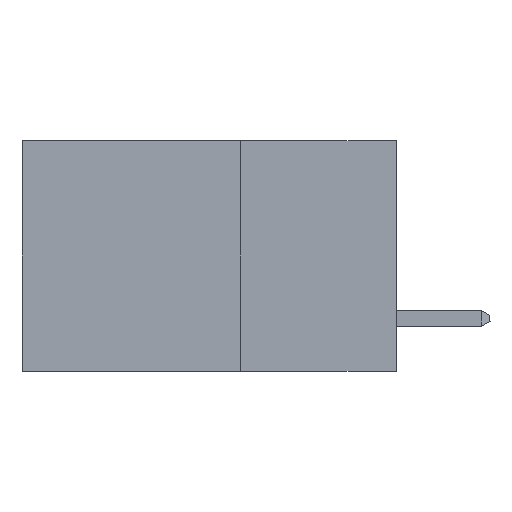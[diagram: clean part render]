
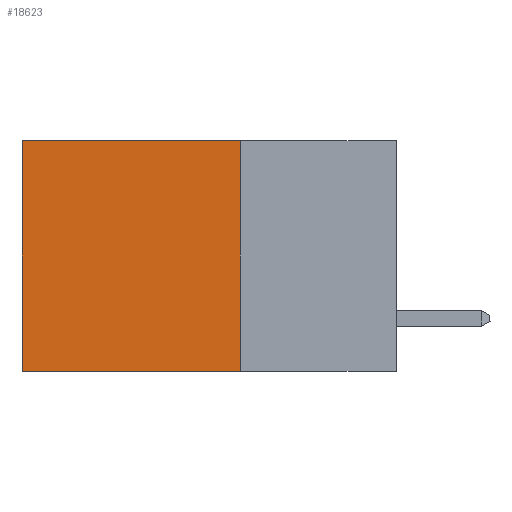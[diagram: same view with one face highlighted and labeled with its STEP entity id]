
A CAD part, left-side view. The second image highlights one B-rep face of the part: STEP entity #18623.
In plain terms, the highlighted planar face has unit normal (-1, 0, 0).
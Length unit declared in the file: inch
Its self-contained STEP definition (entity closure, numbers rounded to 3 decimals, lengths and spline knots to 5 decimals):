
#1898 = LINE ( 'NONE', #2949, #20172 ) ;
#2014 = FACE_OUTER_BOUND ( 'NONE', #14718, .T. ) ;
#2086 = VERTEX_POINT ( 'NONE', #5677 ) ;
#2131 = AXIS2_PLACEMENT_3D ( 'NONE', #17443, #10401, #17752 ) ;
#2949 = CARTESIAN_POINT ( 'NONE',  ( 0.298, 0.25, 0. ) ) ;
#3898 = CARTESIAN_POINT ( 'NONE',  ( 0.298, 0.25, 0. ) ) ;
#4121 = VECTOR ( 'NONE', #18959, 39.37008 ) ;
#4134 = DIRECTION ( 'NONE',  ( 0., 0., -1. ) ) ;
#4562 = CARTESIAN_POINT ( 'NONE',  ( 0.298, 0.6, 0. ) ) ;
#5677 = CARTESIAN_POINT ( 'NONE',  ( 0.298, 0.6, -0.37 ) ) ;
#6279 = DIRECTION ( 'NONE',  ( 0., 1., 0. ) ) ;
#6636 = VERTEX_POINT ( 'NONE', #23257 ) ;
#8073 = LINE ( 'NONE', #4562, #4121 ) ;
#10401 = DIRECTION ( 'NONE',  ( 1., 0., 0. ) ) ;
#10539 = ORIENTED_EDGE ( 'NONE', *, *, #16756, .T. ) ;
#11856 = DIRECTION ( 'NONE',  ( 0., 1., 0. ) ) ;
#11952 = ORIENTED_EDGE ( 'NONE', *, *, #21047, .F. ) ;
#12088 = VECTOR ( 'NONE', #4134, 39.37008 ) ;
#12366 = PLANE ( 'NONE',  #2131 ) ;
#12801 = ORIENTED_EDGE ( 'NONE', *, *, #20851, .F. ) ;
#14718 = EDGE_LOOP ( 'NONE', ( #10539, #11952, #12801, #15706 ) ) ;
#15513 = VERTEX_POINT ( 'NONE', #18837 ) ;
#15706 = ORIENTED_EDGE ( 'NONE', *, *, #21801, .T. ) ;
#15800 = CARTESIAN_POINT ( 'NONE',  ( 0.298, 0.25, 0. ) ) ;
#16756 = EDGE_CURVE ( 'NONE', #6636, #2086, #8073, .T. ) ;
#17443 = CARTESIAN_POINT ( 'NONE',  ( 0.298, 0.25, 0. ) ) ;
#17688 = VECTOR ( 'NONE', #6279, 39.37008 ) ;
#17752 = DIRECTION ( 'NONE',  ( 0., 0., -1. ) ) ;
#17957 = LINE ( 'NONE', #3898, #12088 ) ;
#18623 = ADVANCED_FACE ( 'NONE', ( #2014 ), #12366, .F. ) ;
#18837 = CARTESIAN_POINT ( 'NONE',  ( 0.298, 0.25, -0.37 ) ) ;
#18959 = DIRECTION ( 'NONE',  ( 0., 0., -1. ) ) ;
#20172 = VECTOR ( 'NONE', #11856, 39.37008 ) ;
#20189 = LINE ( 'NONE', #22374, #17688 ) ;
#20851 = EDGE_CURVE ( 'NONE', #22938, #15513, #17957, .T. ) ;
#21047 = EDGE_CURVE ( 'NONE', #15513, #2086, #20189, .T. ) ;
#21801 = EDGE_CURVE ( 'NONE', #22938, #6636, #1898, .T. ) ;
#22374 = CARTESIAN_POINT ( 'NONE',  ( 0.298, 0.25, -0.37 ) ) ;
#22938 = VERTEX_POINT ( 'NONE', #15800 ) ;
#23257 = CARTESIAN_POINT ( 'NONE',  ( 0.298, 0.6, 0. ) ) ;
